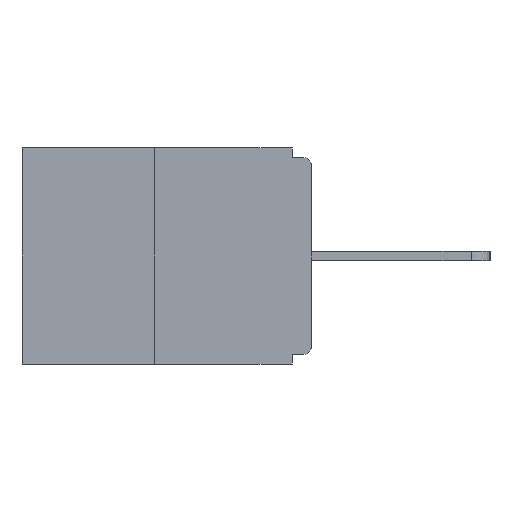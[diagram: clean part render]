
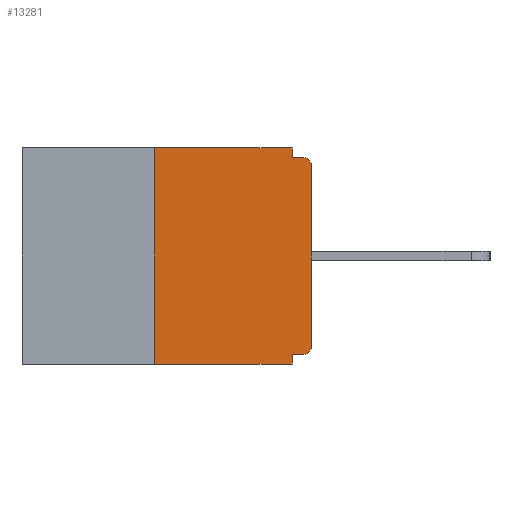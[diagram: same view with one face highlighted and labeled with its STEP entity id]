
A CAD part, left-side view. The second image highlights one B-rep face of the part: STEP entity #13281.
In plain terms, the highlighted planar face has unit normal (-1, 0, 0).
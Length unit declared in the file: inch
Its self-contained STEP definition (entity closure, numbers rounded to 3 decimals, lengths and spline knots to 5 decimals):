
#141 = CARTESIAN_POINT ( 'NONE',  ( 0., 0.031, -0.343 ) ) ;
#520 = CARTESIAN_POINT ( 'NONE',  ( 0., 0.25, 0. ) ) ;
#547 = CARTESIAN_POINT ( 'NONE',  ( 0., 0.46, -0.343 ) ) ;
#1294 = DIRECTION ( 'NONE',  ( 0., 0., -1. ) ) ;
#1769 = DIRECTION ( 'NONE',  ( 0., -1., 0. ) ) ;
#1831 = EDGE_CURVE ( 'NONE', #4556, #5463, #4965, .T. ) ;
#1857 = VERTEX_POINT ( 'NONE', #16043 ) ;
#1870 = ORIENTED_EDGE ( 'NONE', *, *, #5991, .F. ) ;
#1895 = VECTOR ( 'NONE', #1769, 39.37008 ) ;
#2193 = DIRECTION ( 'NONE',  ( 0., 0., -1. ) ) ;
#2215 = EDGE_LOOP ( 'NONE', ( #1870, #7372, #11334, #5910, #16038, #14393, #4505, #11945, #7429, #3254 ) ) ;
#2514 = CARTESIAN_POINT ( 'NONE',  ( 0., 0.015, -0.03 ) ) ;
#2849 = VECTOR ( 'NONE', #3909, 39.37008 ) ;
#2938 = CARTESIAN_POINT ( 'NONE',  ( 0., 0.25, 0. ) ) ;
#3254 = ORIENTED_EDGE ( 'NONE', *, *, #11915, .F. ) ;
#3590 = LINE ( 'NONE', #12419, #14014 ) ;
#3619 = CARTESIAN_POINT ( 'NONE',  ( 0., 0.031, -0.328 ) ) ;
#3764 = AXIS2_PLACEMENT_3D ( 'NONE', #7507, #5963, #10982 ) ;
#3909 = DIRECTION ( 'NONE',  ( 0., 0., -1. ) ) ;
#3984 = DIRECTION ( 'NONE',  ( 0., 1., 0. ) ) ;
#4294 = LINE ( 'NONE', #14364, #9920 ) ;
#4505 = ORIENTED_EDGE ( 'NONE', *, *, #15240, .T. ) ;
#4556 = VERTEX_POINT ( 'NONE', #12801 ) ;
#4857 = VERTEX_POINT ( 'NONE', #3619 ) ;
#4965 = LINE ( 'NONE', #7339, #9254 ) ;
#5213 = CARTESIAN_POINT ( 'NONE',  ( 0., 0.015, -0.015 ) ) ;
#5463 = VERTEX_POINT ( 'NONE', #5213 ) ;
#5517 = VECTOR ( 'NONE', #7885, 39.37008 ) ;
#5518 = LINE ( 'NONE', #15355, #7161 ) ;
#5586 = VERTEX_POINT ( 'NONE', #520 ) ;
#5846 = EDGE_CURVE ( 'NONE', #10350, #4857, #15036, .T. ) ;
#5910 = ORIENTED_EDGE ( 'NONE', *, *, #13026, .F. ) ;
#5952 = CIRCLE ( 'NONE', #14512, 0.015 ) ;
#5963 = DIRECTION ( 'NONE',  ( -1., 0., 0. ) ) ;
#5991 = EDGE_CURVE ( 'NONE', #5586, #15545, #4294, .T. ) ;
#6382 = CARTESIAN_POINT ( 'NONE',  ( 0., 0.46, 0. ) ) ;
#6949 = LINE ( 'NONE', #547, #1895 ) ;
#7156 = EDGE_CURVE ( 'NONE', #1857, #5586, #14057, .T. ) ;
#7161 = VECTOR ( 'NONE', #11668, 39.37008 ) ;
#7262 = DIRECTION ( 'NONE',  ( 0., -1., 0. ) ) ;
#7339 = CARTESIAN_POINT ( 'NONE',  ( 0., 0., -0.015 ) ) ;
#7372 = ORIENTED_EDGE ( 'NONE', *, *, #7156, .F. ) ;
#7429 = ORIENTED_EDGE ( 'NONE', *, *, #1831, .F. ) ;
#7507 = CARTESIAN_POINT ( 'NONE',  ( 0., 0.015, -0.313 ) ) ;
#7885 = DIRECTION ( 'NONE',  ( 0., 0., 1. ) ) ;
#7963 = VERTEX_POINT ( 'NONE', #13297 ) ;
#8055 = CARTESIAN_POINT ( 'NONE',  ( 0., 0.015, -0.328 ) ) ;
#8252 = EDGE_CURVE ( 'NONE', #1857, #12558, #6949, .T. ) ;
#8533 = DIRECTION ( 'NONE',  ( 0., 0., 1. ) ) ;
#8897 = PLANE ( 'NONE',  #9054 ) ;
#9054 = AXIS2_PLACEMENT_3D ( 'NONE', #6382, #9791, #1294 ) ;
#9198 = CIRCLE ( 'NONE', #3764, 0.015 ) ;
#9254 = VECTOR ( 'NONE', #7262, 39.37008 ) ;
#9791 = DIRECTION ( 'NONE',  ( 1., 0., 0. ) ) ;
#9920 = VECTOR ( 'NONE', #10539, 39.37008 ) ;
#10061 = CARTESIAN_POINT ( 'NONE',  ( 0., 0.031, -0.343 ) ) ;
#10350 = VERTEX_POINT ( 'NONE', #8055 ) ;
#10539 = DIRECTION ( 'NONE',  ( 0., -1., 0. ) ) ;
#10982 = DIRECTION ( 'NONE',  ( 0., 0., -1. ) ) ;
#10997 = FACE_OUTER_BOUND ( 'NONE', #2215, .T. ) ;
#11230 = EDGE_CURVE ( 'NONE', #10350, #11795, #9198, .T. ) ;
#11334 = ORIENTED_EDGE ( 'NONE', *, *, #8252, .T. ) ;
#11668 = DIRECTION ( 'NONE',  ( 0., 0., -1. ) ) ;
#11795 = VERTEX_POINT ( 'NONE', #13822 ) ;
#11915 = EDGE_CURVE ( 'NONE', #15545, #4556, #5518, .T. ) ;
#11945 = ORIENTED_EDGE ( 'NONE', *, *, #14877, .T. ) ;
#12239 = CARTESIAN_POINT ( 'NONE',  ( 0., 0.031, 0. ) ) ;
#12419 = CARTESIAN_POINT ( 'NONE',  ( 0., 0., 0. ) ) ;
#12491 = LINE ( 'NONE', #10061, #2849 ) ;
#12558 = VERTEX_POINT ( 'NONE', #141 ) ;
#12801 = CARTESIAN_POINT ( 'NONE',  ( 0., 0.031, -0.015 ) ) ;
#13026 = EDGE_CURVE ( 'NONE', #4857, #12558, #12491, .T. ) ;
#13281 = ADVANCED_FACE ( 'NONE', ( #10997 ), #8897, .F. ) ;
#13296 = DIRECTION ( 'NONE',  ( -1., 0., 0. ) ) ;
#13297 = CARTESIAN_POINT ( 'NONE',  ( 0., 0., -0.03 ) ) ;
#13822 = CARTESIAN_POINT ( 'NONE',  ( 0., 0., -0.313 ) ) ;
#14014 = VECTOR ( 'NONE', #8533, 39.37008 ) ;
#14057 = LINE ( 'NONE', #2938, #5517 ) ;
#14364 = CARTESIAN_POINT ( 'NONE',  ( 0., 0.46, 0. ) ) ;
#14393 = ORIENTED_EDGE ( 'NONE', *, *, #11230, .T. ) ;
#14512 = AXIS2_PLACEMENT_3D ( 'NONE', #2514, #13296, #2193 ) ;
#14877 = EDGE_CURVE ( 'NONE', #7963, #5463, #5952, .T. ) ;
#15036 = LINE ( 'NONE', #15115, #15852 ) ;
#15115 = CARTESIAN_POINT ( 'NONE',  ( 0., 0., -0.328 ) ) ;
#15240 = EDGE_CURVE ( 'NONE', #11795, #7963, #3590, .T. ) ;
#15355 = CARTESIAN_POINT ( 'NONE',  ( 0., 0.031, 0. ) ) ;
#15545 = VERTEX_POINT ( 'NONE', #12239 ) ;
#15852 = VECTOR ( 'NONE', #3984, 39.37008 ) ;
#16038 = ORIENTED_EDGE ( 'NONE', *, *, #5846, .F. ) ;
#16043 = CARTESIAN_POINT ( 'NONE',  ( 0., 0.25, -0.343 ) ) ;
